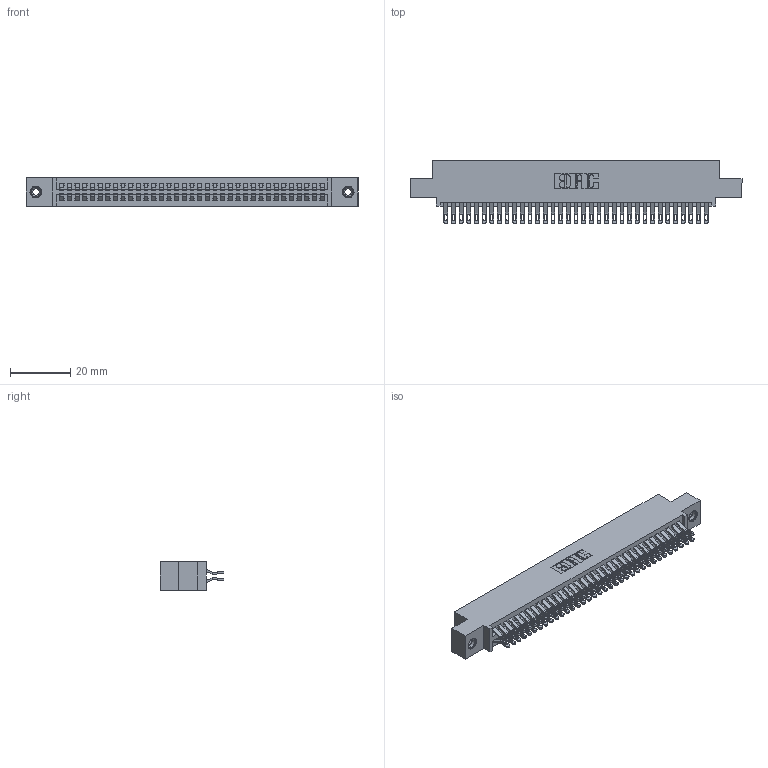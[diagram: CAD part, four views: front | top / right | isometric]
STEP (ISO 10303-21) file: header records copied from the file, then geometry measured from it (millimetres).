
FILE_DESCRIPTION (( 'STEP AP203' ), '1' );
FILE_NAME ('345-070-555-508.STEP', '2018-10-01T09:26:45', ( '' ), ( '' ), 'SwSTEP 2.0', 'SolidWorks 2016', '' );
FILE_SCHEMA (( 'CONFIG_CONTROL_DESIGN' ));
Length unit declared in the file: inch
Products named in the file (4): 345 Part_0.110 Offset - 0.156 Dia-TI; 345-070-555-508; 345-292-001_555 Tail; 345-250-001_345-250-003-102
Assembly tree (73 placements, depth 2):
  345-070-555-508
    345 Part_0.110 Offset - 0.156 Dia-TI
    345-292-001_555 Tail  x70
    345-250-001_345-250-003-102  x2
Bounding box: 110.11 x 21.13 x 9.4 mm (x, y, z)
Volume: 10754.3 mm3; surface area: 16573.5 mm2
Topology: 73 solids, 73 shells, 4110 faces, 12879 edges, 8578 vertices
Faces by surface type: plane 2286, cylinder 1808, cone 12, torus 4
Entity records: 30048 total; most frequent: CARTESIAN_POINT 5061, ORIENTED_EDGE 4958, DIRECTION 4465, EDGE_CURVE 2479, LINE 2167, VECTOR 2167, VERTEX_POINT 1648, AXIS2_PLACEMENT_3D 1149
